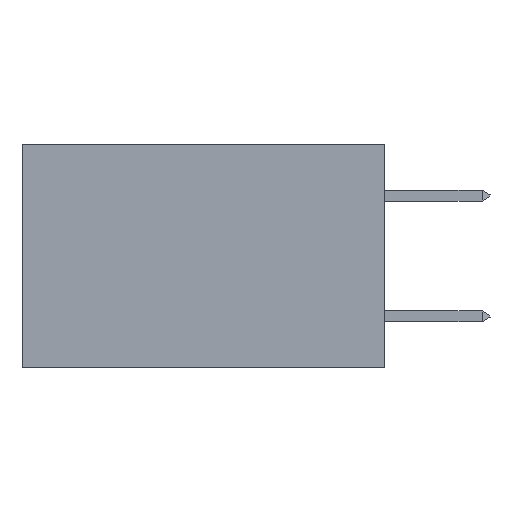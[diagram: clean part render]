
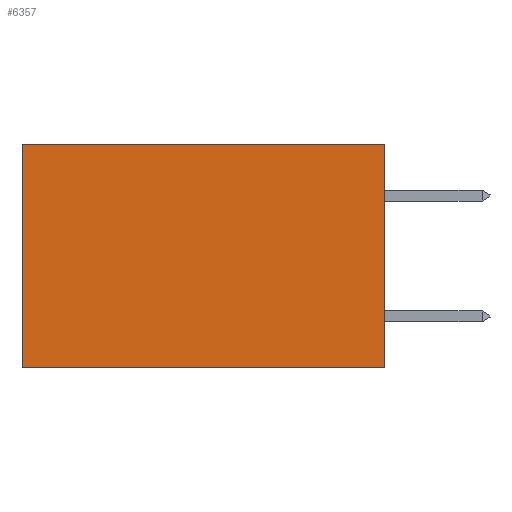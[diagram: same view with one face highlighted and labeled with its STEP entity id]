
A CAD part, left-side view. The second image highlights one B-rep face of the part: STEP entity #6357.
In plain terms, the highlighted planar face has unit normal (-1, 0, 0).
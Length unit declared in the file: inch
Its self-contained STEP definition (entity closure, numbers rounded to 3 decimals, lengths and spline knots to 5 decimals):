
#113 = CARTESIAN_POINT ( 'NONE',  ( 0.2875, 0., -0.37 ) ) ;
#1479 = CARTESIAN_POINT ( 'NONE',  ( 0.2875, 0., 0. ) ) ;
#2713 = VERTEX_POINT ( 'NONE', #33070 ) ;
#2730 = VERTEX_POINT ( 'NONE', #21361 ) ;
#4660 = ORIENTED_EDGE ( 'NONE', *, *, #27944, .T. ) ;
#4833 = DIRECTION ( 'NONE',  ( 0., 0., -1. ) ) ;
#4902 = EDGE_CURVE ( 'NONE', #7830, #2730, #30802, .T. ) ;
#6357 = ADVANCED_FACE ( 'NONE', ( #7653 ), #21155, .F. ) ;
#6756 = CARTESIAN_POINT ( 'NONE',  ( 0.2875, 0., 0. ) ) ;
#7653 = FACE_OUTER_BOUND ( 'NONE', #19910, .T. ) ;
#7830 = VERTEX_POINT ( 'NONE', #36359 ) ;
#9192 = VECTOR ( 'NONE', #30067, 39.37008 ) ;
#9688 = DIRECTION ( 'NONE',  ( 0., 0., -1. ) ) ;
#11025 = LINE ( 'NONE', #36611, #24118 ) ;
#11643 = DIRECTION ( 'NONE',  ( 0., 1., 0. ) ) ;
#11842 = AXIS2_PLACEMENT_3D ( 'NONE', #6756, #27004, #9688 ) ;
#11908 = LINE ( 'NONE', #15902, #9192 ) ;
#14427 = CARTESIAN_POINT ( 'NONE',  ( 0.2875, 0.6, 0. ) ) ;
#15235 = EDGE_CURVE ( 'NONE', #16836, #2730, #11908, .T. ) ;
#15902 = CARTESIAN_POINT ( 'NONE',  ( 0.2875, 0.6, 0. ) ) ;
#16836 = VERTEX_POINT ( 'NONE', #14427 ) ;
#17087 = ORIENTED_EDGE ( 'NONE', *, *, #4902, .F. ) ;
#19910 = EDGE_LOOP ( 'NONE', ( #26646, #17087, #33663, #4660 ) ) ;
#21155 = PLANE ( 'NONE',  #11842 ) ;
#21361 = CARTESIAN_POINT ( 'NONE',  ( 0.2875, 0.6, -0.37 ) ) ;
#23618 = VECTOR ( 'NONE', #27429, 39.37008 ) ;
#24118 = VECTOR ( 'NONE', #4833, 39.37008 ) ;
#26646 = ORIENTED_EDGE ( 'NONE', *, *, #15235, .T. ) ;
#27004 = DIRECTION ( 'NONE',  ( 1., 0., 0. ) ) ;
#27306 = EDGE_CURVE ( 'NONE', #2713, #7830, #11025, .T. ) ;
#27429 = DIRECTION ( 'NONE',  ( 0., 1., 0. ) ) ;
#27944 = EDGE_CURVE ( 'NONE', #2713, #16836, #31273, .T. ) ;
#29907 = VECTOR ( 'NONE', #11643, 39.37008 ) ;
#30067 = DIRECTION ( 'NONE',  ( 0., 0., -1. ) ) ;
#30802 = LINE ( 'NONE', #113, #29907 ) ;
#31273 = LINE ( 'NONE', #1479, #23618 ) ;
#33070 = CARTESIAN_POINT ( 'NONE',  ( 0.2875, 0., 0. ) ) ;
#33663 = ORIENTED_EDGE ( 'NONE', *, *, #27306, .F. ) ;
#36359 = CARTESIAN_POINT ( 'NONE',  ( 0.2875, 0., -0.37 ) ) ;
#36611 = CARTESIAN_POINT ( 'NONE',  ( 0.2875, 0., 0. ) ) ;
